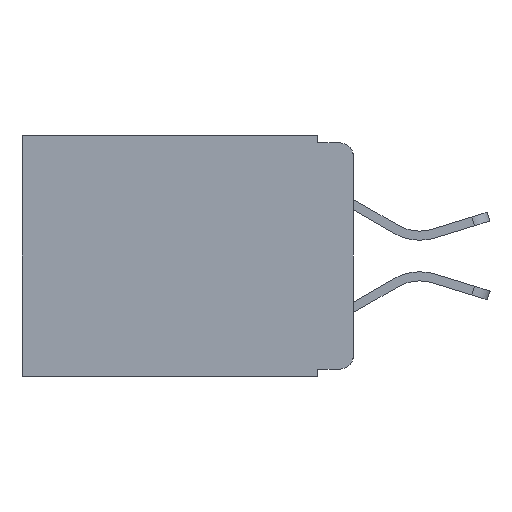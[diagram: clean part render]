
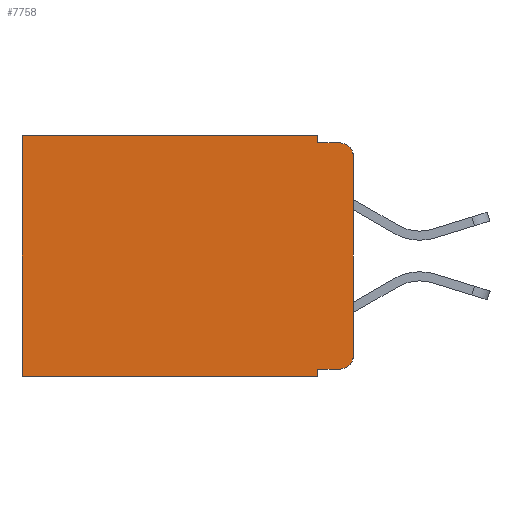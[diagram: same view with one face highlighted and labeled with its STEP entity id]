
A CAD part, left-side view. The second image highlights one B-rep face of the part: STEP entity #7758.
In plain terms, the highlighted planar face has unit normal (-1, 0, 0).
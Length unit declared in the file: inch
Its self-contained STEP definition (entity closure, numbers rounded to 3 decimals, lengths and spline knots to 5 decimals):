
#24 = ORIENTED_EDGE ( 'NONE', *, *, #8732, .F. ) ;
#33 = VERTEX_POINT ( 'NONE', #7120 ) ;
#187 = VERTEX_POINT ( 'NONE', #5272 ) ;
#239 = VECTOR ( 'NONE', #1525, 39.37008 ) ;
#383 = VERTEX_POINT ( 'NONE', #8948 ) ;
#480 = CARTESIAN_POINT ( 'NONE',  ( 0.298, 0., 0. ) ) ;
#504 = VECTOR ( 'NONE', #8790, 39.37008 ) ;
#823 = EDGE_CURVE ( 'NONE', #9022, #7877, #4136, .T. ) ;
#1065 = ORIENTED_EDGE ( 'NONE', *, *, #7501, .T. ) ;
#1233 = ORIENTED_EDGE ( 'NONE', *, *, #4726, .F. ) ;
#1342 = LINE ( 'NONE', #7590, #4286 ) ;
#1412 = DIRECTION ( 'NONE',  ( 0., 0., -1. ) ) ;
#1463 = CARTESIAN_POINT ( 'NONE',  ( 0.298, 0.473, -0.343 ) ) ;
#1525 = DIRECTION ( 'NONE',  ( 0., 0., -1. ) ) ;
#1685 = EDGE_CURVE ( 'NONE', #9605, #9896, #3326, .T. ) ;
#2113 = PLANE ( 'NONE',  #5503 ) ;
#2136 = DIRECTION ( 'NONE',  ( 0., 1., 0. ) ) ;
#2225 = EDGE_CURVE ( 'NONE', #187, #7938, #7350, .T. ) ;
#2229 = DIRECTION ( 'NONE',  ( 0., -1., 0. ) ) ;
#2240 = ORIENTED_EDGE ( 'NONE', *, *, #2695, .T. ) ;
#2321 = CARTESIAN_POINT ( 'NONE',  ( 0.298, 0.473, 0. ) ) ;
#2391 = CARTESIAN_POINT ( 'NONE',  ( 0.298, 0., 0. ) ) ;
#2562 = AXIS2_PLACEMENT_3D ( 'NONE', #7795, #4534, #10026 ) ;
#2695 = EDGE_CURVE ( 'NONE', #9605, #33, #6917, .T. ) ;
#2740 = VERTEX_POINT ( 'NONE', #4494 ) ;
#3077 = DIRECTION ( 'NONE',  ( 0., -1., 0. ) ) ;
#3290 = CARTESIAN_POINT ( 'NONE',  ( 0.298, 0., -0.313 ) ) ;
#3326 = LINE ( 'NONE', #2391, #6455 ) ;
#3354 = VECTOR ( 'NONE', #2229, 39.37008 ) ;
#3646 = VECTOR ( 'NONE', #2136, 39.37008 ) ;
#4102 = VECTOR ( 'NONE', #8103, 39.37008 ) ;
#4136 = LINE ( 'NONE', #4191, #4102 ) ;
#4191 = CARTESIAN_POINT ( 'NONE',  ( 0.298, 0., -0.343 ) ) ;
#4286 = VECTOR ( 'NONE', #4539, 39.37008 ) ;
#4451 = FACE_OUTER_BOUND ( 'NONE', #6269, .T. ) ;
#4494 = CARTESIAN_POINT ( 'NONE',  ( 0.298, 0.473, 0. ) ) ;
#4529 = ORIENTED_EDGE ( 'NONE', *, *, #1685, .F. ) ;
#4534 = DIRECTION ( 'NONE',  ( -1., 0., 0. ) ) ;
#4539 = DIRECTION ( 'NONE',  ( 0., 0., -1. ) ) ;
#4726 = EDGE_CURVE ( 'NONE', #7938, #33, #7882, .T. ) ;
#4831 = CARTESIAN_POINT ( 'NONE',  ( 0.298, 0.051, 0. ) ) ;
#4846 = ORIENTED_EDGE ( 'NONE', *, *, #5707, .T. ) ;
#5167 = DIRECTION ( 'NONE',  ( -1., 0., 0. ) ) ;
#5169 = VECTOR ( 'NONE', #3077, 39.37008 ) ;
#5184 = CARTESIAN_POINT ( 'NONE',  ( 0.298, 0., -0.03 ) ) ;
#5265 = ORIENTED_EDGE ( 'NONE', *, *, #6865, .T. ) ;
#5272 = CARTESIAN_POINT ( 'NONE',  ( 0.298, 0.051, 0. ) ) ;
#5277 = DIRECTION ( 'NONE',  ( 0., 0., -1. ) ) ;
#5398 = CARTESIAN_POINT ( 'NONE',  ( 0.298, 0.02, -0.333 ) ) ;
#5496 = LINE ( 'NONE', #2321, #239 ) ;
#5503 = AXIS2_PLACEMENT_3D ( 'NONE', #9230, #8571, #1412 ) ;
#5707 = EDGE_CURVE ( 'NONE', #187, #2740, #7742, .T. ) ;
#5778 = DIRECTION ( 'NONE',  ( 0., 0., -1. ) ) ;
#6076 = CARTESIAN_POINT ( 'NONE',  ( 0.298, 0.051, -0.333 ) ) ;
#6269 = EDGE_LOOP ( 'NONE', ( #4529, #2240, #1233, #6338, #4846, #1065, #8284, #24, #9073, #5265 ) ) ;
#6338 = ORIENTED_EDGE ( 'NONE', *, *, #2225, .F. ) ;
#6455 = VECTOR ( 'NONE', #5778, 39.37008 ) ;
#6504 = CARTESIAN_POINT ( 'NONE',  ( 0.298, 0.051, -0.343 ) ) ;
#6865 = EDGE_CURVE ( 'NONE', #9673, #9896, #7081, .T. ) ;
#6917 = CIRCLE ( 'NONE', #7715, 0.02 ) ;
#7081 = CIRCLE ( 'NONE', #2562, 0.02 ) ;
#7120 = CARTESIAN_POINT ( 'NONE',  ( 0.298, 0.02, -0.01 ) ) ;
#7231 = EDGE_CURVE ( 'NONE', #383, #9673, #7616, .T. ) ;
#7350 = LINE ( 'NONE', #4831, #504 ) ;
#7501 = EDGE_CURVE ( 'NONE', #2740, #7877, #5496, .T. ) ;
#7590 = CARTESIAN_POINT ( 'NONE',  ( 0.298, 0.051, 0. ) ) ;
#7616 = LINE ( 'NONE', #6076, #3354 ) ;
#7715 = AXIS2_PLACEMENT_3D ( 'NONE', #9118, #5167, #5277 ) ;
#7742 = LINE ( 'NONE', #480, #3646 ) ;
#7758 = ADVANCED_FACE ( 'NONE', ( #4451 ), #2113, .F. ) ;
#7795 = CARTESIAN_POINT ( 'NONE',  ( 0.298, 0.02, -0.313 ) ) ;
#7877 = VERTEX_POINT ( 'NONE', #1463 ) ;
#7882 = LINE ( 'NONE', #10156, #5169 ) ;
#7938 = VERTEX_POINT ( 'NONE', #9775 ) ;
#8103 = DIRECTION ( 'NONE',  ( 0., 1., 0. ) ) ;
#8284 = ORIENTED_EDGE ( 'NONE', *, *, #823, .F. ) ;
#8571 = DIRECTION ( 'NONE',  ( 1., 0., 0. ) ) ;
#8732 = EDGE_CURVE ( 'NONE', #383, #9022, #1342, .T. ) ;
#8790 = DIRECTION ( 'NONE',  ( 0., 0., -1. ) ) ;
#8948 = CARTESIAN_POINT ( 'NONE',  ( 0.298, 0.051, -0.333 ) ) ;
#9022 = VERTEX_POINT ( 'NONE', #6504 ) ;
#9073 = ORIENTED_EDGE ( 'NONE', *, *, #7231, .T. ) ;
#9118 = CARTESIAN_POINT ( 'NONE',  ( 0.298, 0.02, -0.03 ) ) ;
#9230 = CARTESIAN_POINT ( 'NONE',  ( 0.298, 0., 0. ) ) ;
#9605 = VERTEX_POINT ( 'NONE', #5184 ) ;
#9673 = VERTEX_POINT ( 'NONE', #5398 ) ;
#9775 = CARTESIAN_POINT ( 'NONE',  ( 0.298, 0.051, -0.01 ) ) ;
#9896 = VERTEX_POINT ( 'NONE', #3290 ) ;
#10026 = DIRECTION ( 'NONE',  ( 0., 0., -1. ) ) ;
#10156 = CARTESIAN_POINT ( 'NONE',  ( 0.298, 0.051, -0.01 ) ) ;
